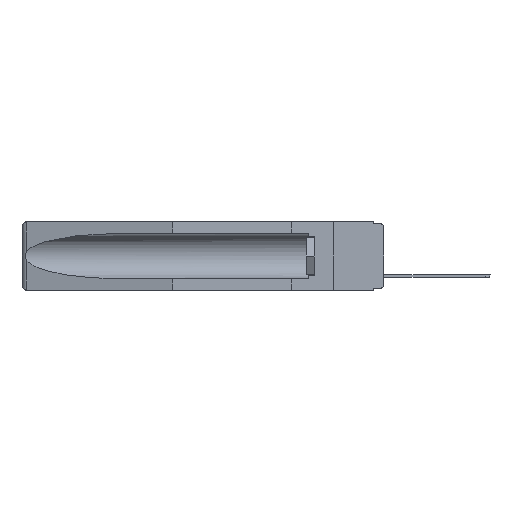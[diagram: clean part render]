
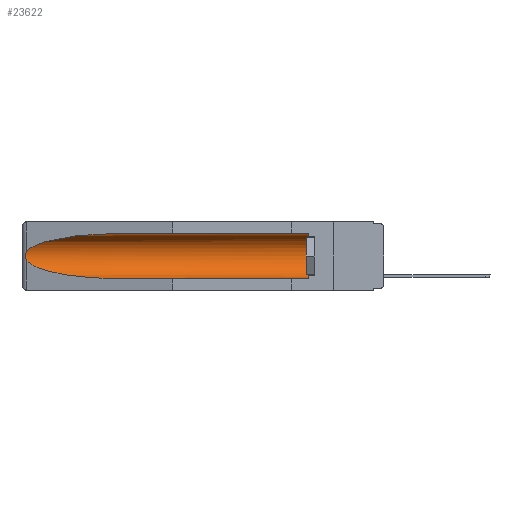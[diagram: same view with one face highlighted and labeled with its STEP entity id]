
A CAD part, left-side view. The second image highlights one B-rep face of the part: STEP entity #23622.
In plain terms, the highlighted cylindrical face has radius 2.857 mm (diameter 5.715 mm), a partial arc.
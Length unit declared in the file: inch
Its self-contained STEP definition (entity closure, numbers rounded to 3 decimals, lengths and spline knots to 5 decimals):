
#833 = ORIENTED_EDGE ( 'NONE', *, *, #1433, .T. ) ;
#1256 = ORIENTED_EDGE ( 'NONE', *, *, #10571, .F. ) ;
#1433 = EDGE_CURVE ( 'NONE', #12730, #12241, #2772, .T. ) ;
#1493 = DIRECTION ( 'NONE',  ( 0., 0., 1. ) ) ;
#1821 = CARTESIAN_POINT ( 'NONE',  ( 0.26537, 1.52718, -0.19328 ) ) ;
#1946 = CARTESIAN_POINT ( 'NONE',  ( 0.26597, 1.5296, -0.19026 ) ) ;
#2745 = DIRECTION ( 'NONE',  ( 0., -1., 0. ) ) ;
#2772 = LINE ( 'NONE', #18042, #2775 ) ;
#2775 = VECTOR ( 'NONE', #23473, 39.37008 ) ;
#2840 = CARTESIAN_POINT ( 'NONE',  ( 0.155, 0.126, -0.284 ) ) ;
#2860 = ORIENTED_EDGE ( 'NONE', *, *, #16742, .T. ) ;
#3814 = CARTESIAN_POINT ( 'NONE',  ( 0.2675, 1.53308, -0.16763 ) ) ;
#3826 = CARTESIAN_POINT ( 'NONE',  ( 0.26537, 1.52718, -0.19328 ) ) ;
#5252 = CYLINDRICAL_SURFACE ( 'NONE', #16186, 0.1125 ) ;
#6348 = VERTEX_POINT ( 'NONE', #2840 ) ;
#7182 = CARTESIAN_POINT ( 'NONE',  ( 0.26597, 1.52961, -0.15275 ) ) ;
#7296 = CARTESIAN_POINT ( 'NONE',  ( 0.26537, 1.52718, -0.14972 ) ) ;
#7426 = VECTOR ( 'NONE', #14062, 39.37008 ) ;
#7629 = ORIENTED_EDGE ( 'NONE', *, *, #10420, .T. ) ;
#9021 = CARTESIAN_POINT ( 'NONE',  ( 0.155, 1.07973, -0.284 ) ) ;
#9117 =( BOUNDED_CURVE ( )  B_SPLINE_CURVE ( 3, ( #24255, #20419, #17420, #7296 ),
 .UNSPECIFIED., .F., .F. ) 
 B_SPLINE_CURVE_WITH_KNOTS ( ( 4, 4 ),
 ( 4.71239, 6.08839 ),
 .UNSPECIFIED. ) 
 CURVE ( )  GEOMETRIC_REPRESENTATION_ITEM ( )  RATIONAL_B_SPLINE_CURVE ( ( 1., 0.848, 0.848, 1. ) ) 
 REPRESENTATION_ITEM ( '' )  );
#9156 = CARTESIAN_POINT ( 'NONE',  ( 0.25451, 1.48313, -0.24835 ) ) ;
#9288 = CARTESIAN_POINT ( 'NONE',  ( 0.21114, 1.30732, -0.284 ) ) ;
#9417 = CARTESIAN_POINT ( 'NONE',  ( 0.2673, 1.5327, -0.16383 ) ) ;
#9763 =( BOUNDED_CURVE ( )  B_SPLINE_CURVE ( 3, ( #1821, #9156, #9288, #9021 ),
 .UNSPECIFIED., .F., .F. ) 
 B_SPLINE_CURVE_WITH_KNOTS ( ( 4, 4 ),
 ( 0.1948, 1.5708 ),
 .UNSPECIFIED. ) 
 CURVE ( )  GEOMETRIC_REPRESENTATION_ITEM ( )  RATIONAL_B_SPLINE_CURVE ( ( 1., 0.848, 0.848, 1. ) ) 
 REPRESENTATION_ITEM ( '' )  );
#10366 = EDGE_CURVE ( 'NONE', #20197, #10974, #9763, .T. ) ;
#10420 = EDGE_CURVE ( 'NONE', #12241, #16551, #9117, .T. ) ;
#10571 = EDGE_CURVE ( 'NONE', #6348, #10974, #23462, .T. ) ;
#10717 = CARTESIAN_POINT ( 'NONE',  ( 0.155, -0.30754, -0.1715 ) ) ;
#10974 = VERTEX_POINT ( 'NONE', #12582 ) ;
#11267 = CARTESIAN_POINT ( 'NONE',  ( 0.2673, 1.53269, -0.17917 ) ) ;
#11378 = CARTESIAN_POINT ( 'NONE',  ( 0.26655, 1.53094, -0.18657 ) ) ;
#12236 = ORIENTED_EDGE ( 'NONE', *, *, #10366, .T. ) ;
#12241 = VERTEX_POINT ( 'NONE', #16941 ) ;
#12582 = CARTESIAN_POINT ( 'NONE',  ( 0.155, 1.07973, -0.284 ) ) ;
#12592 = DIRECTION ( 'NONE',  ( 0., 0., 1. ) ) ;
#12730 = VERTEX_POINT ( 'NONE', #19229 ) ;
#12766 = CARTESIAN_POINT ( 'NONE',  ( 0.26537, 1.52718, -0.14972 ) ) ;
#12842 = DIRECTION ( 'NONE',  ( 0., 1., 0. ) ) ;
#13131 = CARTESIAN_POINT ( 'NONE',  ( 0.2675, 1.53308, -0.17534 ) ) ;
#13223 = CIRCLE ( 'NONE', #17161, 0.1125 ) ;
#14062 = DIRECTION ( 'NONE',  ( 0., 1., 0. ) ) ;
#14718 = B_SPLINE_CURVE_WITH_KNOTS ( 'NONE', 3,
 ( #24260, #7182, #14752, #9417, #3814, #13131, #11267, #11378, #1946, #18826 ),
 .UNSPECIFIED., .F., .F.,
 ( 4, 2, 2, 2, 4 ),
 ( 0., 0.00029, 0.00058, 0.00087, 0.00117 ),
 .UNSPECIFIED. ) ;
#14752 = CARTESIAN_POINT ( 'NONE',  ( 0.26654, 1.53092, -0.15636 ) ) ;
#16186 = AXIS2_PLACEMENT_3D ( 'NONE', #10717, #12842, #12592 ) ;
#16551 = VERTEX_POINT ( 'NONE', #12766 ) ;
#16742 = EDGE_CURVE ( 'NONE', #16551, #20197, #14718, .T. ) ;
#16941 = CARTESIAN_POINT ( 'NONE',  ( 0.155, 1.07973, -0.059 ) ) ;
#17161 = AXIS2_PLACEMENT_3D ( 'NONE', #19733, #2745, #1493 ) ;
#17168 = ORIENTED_EDGE ( 'NONE', *, *, #19592, .T. ) ;
#17420 = CARTESIAN_POINT ( 'NONE',  ( 0.25451, 1.48313, -0.09465 ) ) ;
#18042 = CARTESIAN_POINT ( 'NONE',  ( 0.155, -0.30754, -0.059 ) ) ;
#18826 = CARTESIAN_POINT ( 'NONE',  ( 0.26537, 1.52718, -0.19328 ) ) ;
#19229 = CARTESIAN_POINT ( 'NONE',  ( 0.155, 0.126, -0.059 ) ) ;
#19332 = EDGE_LOOP ( 'NONE', ( #7629, #2860, #12236, #1256, #17168, #833 ) ) ;
#19592 = EDGE_CURVE ( 'NONE', #6348, #12730, #13223, .T. ) ;
#19733 = CARTESIAN_POINT ( 'NONE',  ( 0.155, 0.126, -0.1715 ) ) ;
#20197 = VERTEX_POINT ( 'NONE', #3826 ) ;
#20376 = FACE_OUTER_BOUND ( 'NONE', #19332, .T. ) ;
#20419 = CARTESIAN_POINT ( 'NONE',  ( 0.21114, 1.30732, -0.059 ) ) ;
#21492 = CARTESIAN_POINT ( 'NONE',  ( 0.155, -0.30754, -0.284 ) ) ;
#23462 = LINE ( 'NONE', #21492, #7426 ) ;
#23473 = DIRECTION ( 'NONE',  ( 0., 1., 0. ) ) ;
#23622 = ADVANCED_FACE ( 'NONE', ( #20376 ), #5252, .F. ) ;
#24255 = CARTESIAN_POINT ( 'NONE',  ( 0.155, 1.07973, -0.059 ) ) ;
#24260 = CARTESIAN_POINT ( 'NONE',  ( 0.26537, 1.52718, -0.14972 ) ) ;
